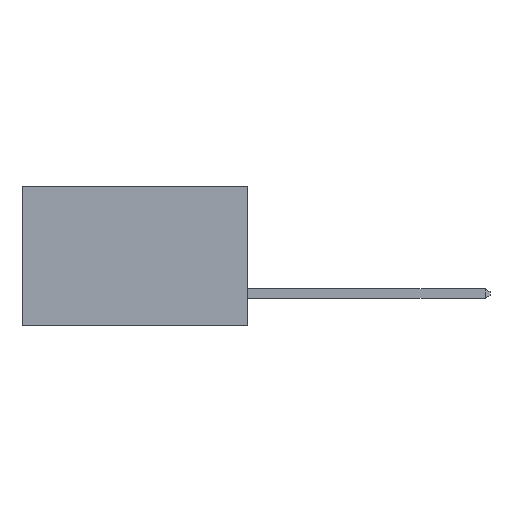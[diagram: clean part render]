
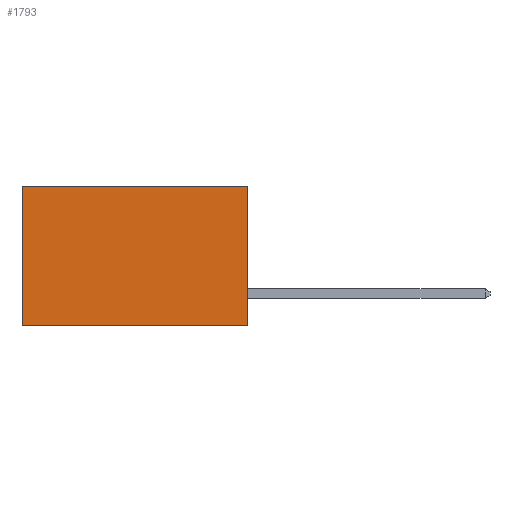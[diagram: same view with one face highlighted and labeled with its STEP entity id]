
A CAD part, left-side view. The second image highlights one B-rep face of the part: STEP entity #1793.
In plain terms, the highlighted planar face has unit normal (-1, 0, 0).
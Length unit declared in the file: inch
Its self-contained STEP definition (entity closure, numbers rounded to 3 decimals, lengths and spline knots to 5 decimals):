
#647 = LINE ( 'NONE', #2475, #9880 ) ;
#885 = LINE ( 'NONE', #6028, #10056 ) ;
#947 = ORIENTED_EDGE ( 'NONE', *, *, #1903, .T. ) ;
#1037 = EDGE_CURVE ( 'NONE', #7672, #2429, #11443, .T. ) ;
#1793 = ADVANCED_FACE ( 'NONE', ( #7534 ), #8569, .F. ) ;
#1903 = EDGE_CURVE ( 'NONE', #3163, #4013, #885, .T. ) ;
#2429 = VERTEX_POINT ( 'NONE', #3666 ) ;
#2475 = CARTESIAN_POINT ( 'NONE',  ( 0.2615, 0., -0.37 ) ) ;
#2632 = LINE ( 'NONE', #9169, #9393 ) ;
#3163 = VERTEX_POINT ( 'NONE', #6893 ) ;
#3464 = DIRECTION ( 'NONE',  ( 0., 0., -1. ) ) ;
#3489 = ORIENTED_EDGE ( 'NONE', *, *, #7261, .F. ) ;
#3666 = CARTESIAN_POINT ( 'NONE',  ( 0.2615, 0., -0.37 ) ) ;
#3861 = CARTESIAN_POINT ( 'NONE',  ( 0.2615, 0., 0. ) ) ;
#4013 = VERTEX_POINT ( 'NONE', #7100 ) ;
#5978 = ORIENTED_EDGE ( 'NONE', *, *, #1037, .F. ) ;
#6028 = CARTESIAN_POINT ( 'NONE',  ( 0.2615, 0.6, -0.37 ) ) ;
#6821 = EDGE_CURVE ( 'NONE', #7672, #3163, #2632, .T. ) ;
#6893 = CARTESIAN_POINT ( 'NONE',  ( 0.2615, 0.6, 0. ) ) ;
#7100 = CARTESIAN_POINT ( 'NONE',  ( 0.2615, 0.6, -0.37 ) ) ;
#7261 = EDGE_CURVE ( 'NONE', #2429, #4013, #647, .T. ) ;
#7349 = AXIS2_PLACEMENT_3D ( 'NONE', #10113, #8676, #8955 ) ;
#7534 = FACE_OUTER_BOUND ( 'NONE', #9986, .T. ) ;
#7672 = VERTEX_POINT ( 'NONE', #3861 ) ;
#8255 = ORIENTED_EDGE ( 'NONE', *, *, #6821, .T. ) ;
#8569 = PLANE ( 'NONE',  #7349 ) ;
#8676 = DIRECTION ( 'NONE',  ( 1., 0., 0. ) ) ;
#8955 = DIRECTION ( 'NONE',  ( 0., 0., -1. ) ) ;
#9169 = CARTESIAN_POINT ( 'NONE',  ( 0.2615, 0., 0. ) ) ;
#9347 = VECTOR ( 'NONE', #10876, 39.37008 ) ;
#9393 = VECTOR ( 'NONE', #9954, 39.37008 ) ;
#9535 = DIRECTION ( 'NONE',  ( 0., 1., 0. ) ) ;
#9880 = VECTOR ( 'NONE', #9535, 39.37008 ) ;
#9881 = CARTESIAN_POINT ( 'NONE',  ( 0.2615, 0., -0.37 ) ) ;
#9954 = DIRECTION ( 'NONE',  ( 0., 1., 0. ) ) ;
#9986 = EDGE_LOOP ( 'NONE', ( #947, #3489, #5978, #8255 ) ) ;
#10056 = VECTOR ( 'NONE', #3464, 39.37008 ) ;
#10113 = CARTESIAN_POINT ( 'NONE',  ( 0.2615, 0., -0.37 ) ) ;
#10876 = DIRECTION ( 'NONE',  ( 0., 0., -1. ) ) ;
#11443 = LINE ( 'NONE', #9881, #9347 ) ;
